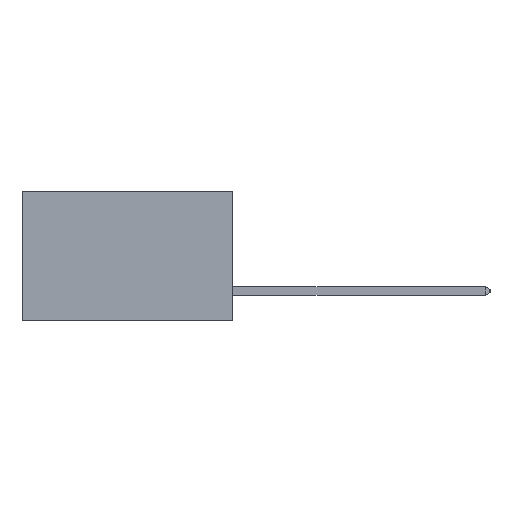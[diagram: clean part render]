
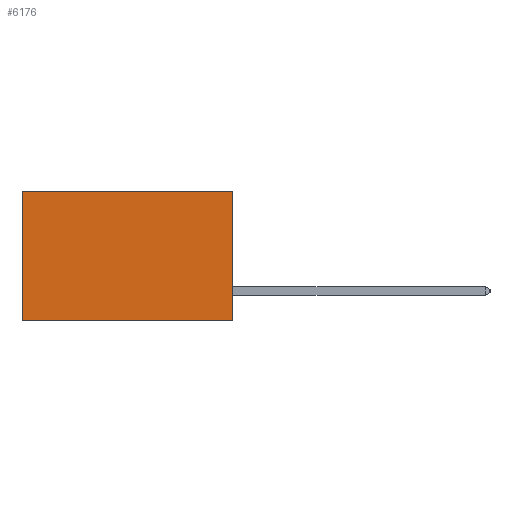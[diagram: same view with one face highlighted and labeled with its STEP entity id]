
A CAD part, left-side view. The second image highlights one B-rep face of the part: STEP entity #6176.
In plain terms, the highlighted planar face has unit normal (-1, 0, 0).
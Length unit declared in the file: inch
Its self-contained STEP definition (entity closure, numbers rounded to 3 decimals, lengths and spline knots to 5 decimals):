
#501 = EDGE_LOOP ( 'NONE', ( #4244, #3606, #5866, #7640 ) ) ;
#1377 = CARTESIAN_POINT ( 'NONE',  ( 0.2875, 0.6, -0.37 ) ) ;
#1549 = CARTESIAN_POINT ( 'NONE',  ( 0.2875, 0., 0. ) ) ;
#2046 = VECTOR ( 'NONE', #8976, 39.37008 ) ;
#2129 = FACE_OUTER_BOUND ( 'NONE', #501, .T. ) ;
#2143 = PLANE ( 'NONE',  #11483 ) ;
#3173 = DIRECTION ( 'NONE',  ( 0., 0., -1. ) ) ;
#3335 = VECTOR ( 'NONE', #5019, 39.37008 ) ;
#3426 = VERTEX_POINT ( 'NONE', #10938 ) ;
#3432 = EDGE_CURVE ( 'NONE', #3426, #4490, #9751, .T. ) ;
#3540 = EDGE_CURVE ( 'NONE', #4490, #10576, #4063, .T. ) ;
#3606 = ORIENTED_EDGE ( 'NONE', *, *, #8613, .F. ) ;
#3743 = VECTOR ( 'NONE', #3173, 39.37008 ) ;
#4063 = LINE ( 'NONE', #5847, #3743 ) ;
#4102 = VECTOR ( 'NONE', #9029, 39.37008 ) ;
#4244 = ORIENTED_EDGE ( 'NONE', *, *, #3540, .T. ) ;
#4490 = VERTEX_POINT ( 'NONE', #10953 ) ;
#5019 = DIRECTION ( 'NONE',  ( 0., 1., 0. ) ) ;
#5107 = DIRECTION ( 'NONE',  ( 1., 0., 0. ) ) ;
#5847 = CARTESIAN_POINT ( 'NONE',  ( 0.2875, 0.6, 0. ) ) ;
#5866 = ORIENTED_EDGE ( 'NONE', *, *, #9670, .F. ) ;
#6176 = ADVANCED_FACE ( 'NONE', ( #2129 ), #2143, .F. ) ;
#6733 = CARTESIAN_POINT ( 'NONE',  ( 0.2875, 0., 0. ) ) ;
#7640 = ORIENTED_EDGE ( 'NONE', *, *, #3432, .T. ) ;
#8363 = LINE ( 'NONE', #1549, #4102 ) ;
#8613 = EDGE_CURVE ( 'NONE', #9594, #10576, #11872, .T. ) ;
#8976 = DIRECTION ( 'NONE',  ( 0., 1., 0. ) ) ;
#9029 = DIRECTION ( 'NONE',  ( 0., 0., -1. ) ) ;
#9594 = VERTEX_POINT ( 'NONE', #11612 ) ;
#9670 = EDGE_CURVE ( 'NONE', #3426, #9594, #8363, .T. ) ;
#9751 = LINE ( 'NONE', #6733, #2046 ) ;
#10489 = CARTESIAN_POINT ( 'NONE',  ( 0.2875, 0., 0. ) ) ;
#10576 = VERTEX_POINT ( 'NONE', #1377 ) ;
#10938 = CARTESIAN_POINT ( 'NONE',  ( 0.2875, 0., 0. ) ) ;
#10953 = CARTESIAN_POINT ( 'NONE',  ( 0.2875, 0.6, 0. ) ) ;
#11289 = CARTESIAN_POINT ( 'NONE',  ( 0.2875, 0., -0.37 ) ) ;
#11369 = DIRECTION ( 'NONE',  ( 0., 0., -1. ) ) ;
#11483 = AXIS2_PLACEMENT_3D ( 'NONE', #10489, #5107, #11369 ) ;
#11612 = CARTESIAN_POINT ( 'NONE',  ( 0.2875, 0., -0.37 ) ) ;
#11872 = LINE ( 'NONE', #11289, #3335 ) ;
